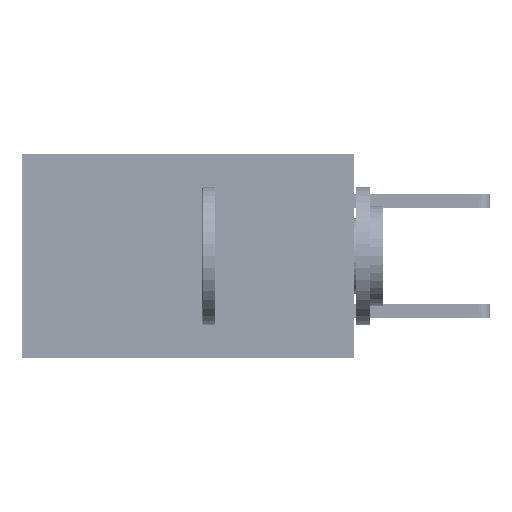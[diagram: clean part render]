
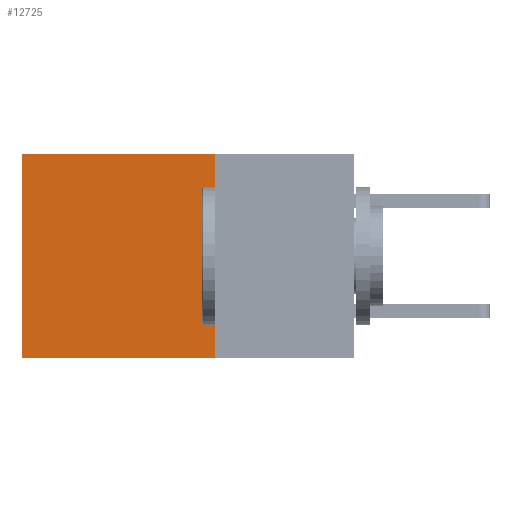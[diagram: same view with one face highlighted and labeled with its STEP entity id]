
A CAD part, left-side view. The second image highlights one B-rep face of the part: STEP entity #12725.
In plain terms, the highlighted planar face has unit normal (-1, 0, 0).
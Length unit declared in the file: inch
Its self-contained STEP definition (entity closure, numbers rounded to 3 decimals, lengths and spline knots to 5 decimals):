
#1346 = DIRECTION ( 'NONE',  ( 0., 0., -1. ) ) ;
#3837 = VECTOR ( 'NONE', #38417, 39.37008 ) ;
#3981 = VERTEX_POINT ( 'NONE', #23768 ) ;
#4383 = ORIENTED_EDGE ( 'NONE', *, *, #16537, .F. ) ;
#4990 = LINE ( 'NONE', #30831, #3837 ) ;
#5321 = CARTESIAN_POINT ( 'NONE',  ( 0.2875, 0.25, -0.37 ) ) ;
#5893 = ORIENTED_EDGE ( 'NONE', *, *, #39607, .F. ) ;
#7319 = VERTEX_POINT ( 'NONE', #5321 ) ;
#11996 = EDGE_CURVE ( 'NONE', #3981, #20096, #4990, .T. ) ;
#12725 = ADVANCED_FACE ( 'NONE', ( #22867 ), #33554, .F. ) ;
#13960 = CARTESIAN_POINT ( 'NONE',  ( 0.2875, 0.6, 0. ) ) ;
#16537 = EDGE_CURVE ( 'NONE', #3981, #7319, #34012, .T. ) ;
#17202 = DIRECTION ( 'NONE',  ( 0., 0., -1. ) ) ;
#19510 = LINE ( 'NONE', #21484, #24742 ) ;
#19600 = CARTESIAN_POINT ( 'NONE',  ( 0.2875, 0.25, 0. ) ) ;
#20096 = VERTEX_POINT ( 'NONE', #22979 ) ;
#21484 = CARTESIAN_POINT ( 'NONE',  ( 0.2875, 0.25, -0.37 ) ) ;
#22867 = FACE_OUTER_BOUND ( 'NONE', #43917, .T. ) ;
#22979 = CARTESIAN_POINT ( 'NONE',  ( 0.2875, 0.6, 0. ) ) ;
#23014 = AXIS2_PLACEMENT_3D ( 'NONE', #19600, #42368, #1346 ) ;
#23017 = LINE ( 'NONE', #13960, #44945 ) ;
#23564 = ORIENTED_EDGE ( 'NONE', *, *, #11996, .T. ) ;
#23768 = CARTESIAN_POINT ( 'NONE',  ( 0.2875, 0.25, 0. ) ) ;
#24163 = VECTOR ( 'NONE', #33625, 39.37008 ) ;
#24742 = VECTOR ( 'NONE', #40050, 39.37008 ) ;
#24795 = ORIENTED_EDGE ( 'NONE', *, *, #32208, .T. ) ;
#27012 = VERTEX_POINT ( 'NONE', #39411 ) ;
#30831 = CARTESIAN_POINT ( 'NONE',  ( 0.2875, 0.25, 0. ) ) ;
#32208 = EDGE_CURVE ( 'NONE', #20096, #27012, #23017, .T. ) ;
#33554 = PLANE ( 'NONE',  #23014 ) ;
#33625 = DIRECTION ( 'NONE',  ( 0., 0., -1. ) ) ;
#34012 = LINE ( 'NONE', #44077, #24163 ) ;
#38417 = DIRECTION ( 'NONE',  ( 0., 1., 0. ) ) ;
#39411 = CARTESIAN_POINT ( 'NONE',  ( 0.2875, 0.6, -0.37 ) ) ;
#39607 = EDGE_CURVE ( 'NONE', #7319, #27012, #19510, .T. ) ;
#40050 = DIRECTION ( 'NONE',  ( 0., 1., 0. ) ) ;
#42368 = DIRECTION ( 'NONE',  ( 1., 0., 0. ) ) ;
#43917 = EDGE_LOOP ( 'NONE', ( #24795, #5893, #4383, #23564 ) ) ;
#44077 = CARTESIAN_POINT ( 'NONE',  ( 0.2875, 0.25, 0. ) ) ;
#44945 = VECTOR ( 'NONE', #17202, 39.37008 ) ;
